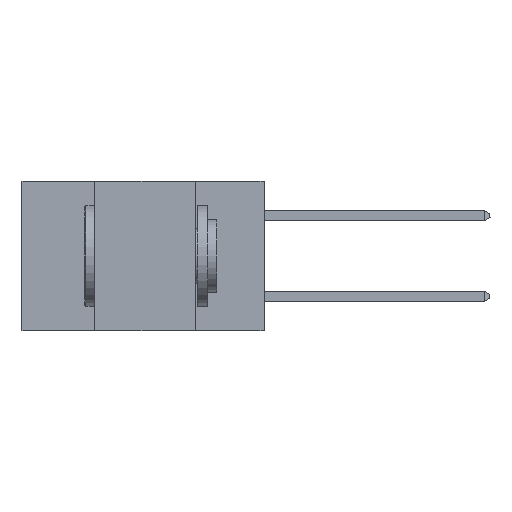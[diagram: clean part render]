
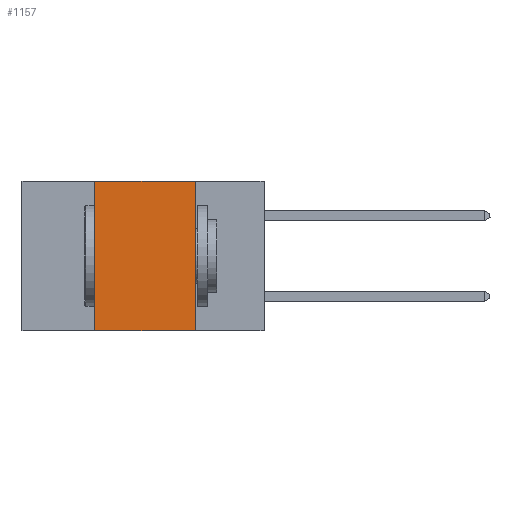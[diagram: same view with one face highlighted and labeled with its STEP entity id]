
A CAD part, left-side view. The second image highlights one B-rep face of the part: STEP entity #1157.
In plain terms, the highlighted planar face has unit normal (-1, 0, 0).
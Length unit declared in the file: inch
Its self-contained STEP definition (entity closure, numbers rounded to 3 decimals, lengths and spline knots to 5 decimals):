
#437 = DIRECTION ( 'NONE',  ( 1., 0., 0. ) ) ;
#778 = VECTOR ( 'NONE', #2553, 39.37008 ) ;
#1157 = ADVANCED_FACE ( 'NONE', ( #8996 ), #19989, .F. ) ;
#2553 = DIRECTION ( 'NONE',  ( 0., 0., -1. ) ) ;
#2711 = CARTESIAN_POINT ( 'NONE',  ( 0., 0.42, -0.37 ) ) ;
#3021 = CARTESIAN_POINT ( 'NONE',  ( 0., 0.17, -0.37 ) ) ;
#4267 = CARTESIAN_POINT ( 'NONE',  ( 0., 0.17, 0. ) ) ;
#4502 = EDGE_CURVE ( 'NONE', #16807, #9704, #20000, .T. ) ;
#4920 = LINE ( 'NONE', #10446, #778 ) ;
#6396 = ORIENTED_EDGE ( 'NONE', *, *, #18979, .T. ) ;
#6774 = AXIS2_PLACEMENT_3D ( 'NONE', #12110, #437, #16346 ) ;
#6917 = ORIENTED_EDGE ( 'NONE', *, *, #10191, .F. ) ;
#8343 = VERTEX_POINT ( 'NONE', #2711 ) ;
#8996 = FACE_OUTER_BOUND ( 'NONE', #25270, .T. ) ;
#9075 = VERTEX_POINT ( 'NONE', #3021 ) ;
#9309 = CARTESIAN_POINT ( 'NONE',  ( 0., 0.42, 0. ) ) ;
#9487 = VECTOR ( 'NONE', #14957, 39.37008 ) ;
#9704 = VERTEX_POINT ( 'NONE', #4267 ) ;
#10191 = EDGE_CURVE ( 'NONE', #8343, #16807, #14369, .T. ) ;
#10446 = CARTESIAN_POINT ( 'NONE',  ( 0., 0.17, 0. ) ) ;
#12110 = CARTESIAN_POINT ( 'NONE',  ( 0., 0.6, 0. ) ) ;
#12949 = DIRECTION ( 'NONE',  ( 0., -1., 0. ) ) ;
#12963 = CARTESIAN_POINT ( 'NONE',  ( 0., 0.6, 0. ) ) ;
#12965 = VECTOR ( 'NONE', #12949, 39.37008 ) ;
#13033 = CARTESIAN_POINT ( 'NONE',  ( 0., 0.6, -0.37 ) ) ;
#13299 = CARTESIAN_POINT ( 'NONE',  ( 0., 0.42, 0. ) ) ;
#13742 = VECTOR ( 'NONE', #15253, 39.37008 ) ;
#13787 = ORIENTED_EDGE ( 'NONE', *, *, #4502, .F. ) ;
#13825 = ORIENTED_EDGE ( 'NONE', *, *, #17200, .F. ) ;
#14369 = LINE ( 'NONE', #9309, #13742 ) ;
#14957 = DIRECTION ( 'NONE',  ( 0., -1., 0. ) ) ;
#15253 = DIRECTION ( 'NONE',  ( 0., 0., 1. ) ) ;
#16346 = DIRECTION ( 'NONE',  ( 0., 0., -1. ) ) ;
#16807 = VERTEX_POINT ( 'NONE', #13299 ) ;
#17200 = EDGE_CURVE ( 'NONE', #9704, #9075, #4920, .T. ) ;
#18979 = EDGE_CURVE ( 'NONE', #8343, #9075, #19152, .T. ) ;
#19152 = LINE ( 'NONE', #13033, #12965 ) ;
#19989 = PLANE ( 'NONE',  #6774 ) ;
#20000 = LINE ( 'NONE', #12963, #9487 ) ;
#25270 = EDGE_LOOP ( 'NONE', ( #13825, #13787, #6917, #6396 ) ) ;
